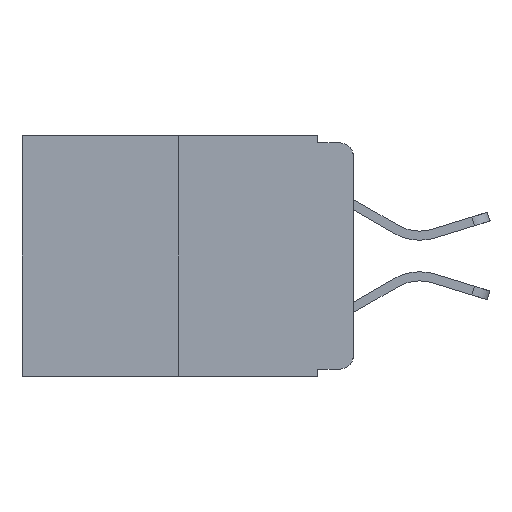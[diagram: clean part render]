
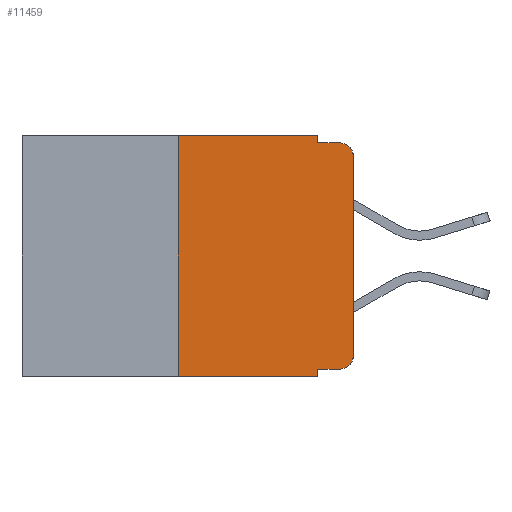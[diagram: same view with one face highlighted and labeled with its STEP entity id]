
A CAD part, left-side view. The second image highlights one B-rep face of the part: STEP entity #11459.
In plain terms, the highlighted planar face has unit normal (-1, 0, 0).
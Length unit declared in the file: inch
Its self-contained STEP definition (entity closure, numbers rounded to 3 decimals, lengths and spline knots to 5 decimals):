
#16 = ORIENTED_EDGE ( 'NONE', *, *, #14934, .T. ) ;
#308 = CARTESIAN_POINT ( 'NONE',  ( 0., 0.473, -0.343 ) ) ;
#484 = VERTEX_POINT ( 'NONE', #1440 ) ;
#561 = ORIENTED_EDGE ( 'NONE', *, *, #11764, .T. ) ;
#625 = VERTEX_POINT ( 'NONE', #16814 ) ;
#957 = VERTEX_POINT ( 'NONE', #11274 ) ;
#1167 = DIRECTION ( 'NONE',  ( 0., -1., 0. ) ) ;
#1254 = DIRECTION ( 'NONE',  ( 0., 0., -1. ) ) ;
#1336 = CARTESIAN_POINT ( 'NONE',  ( 0., 0., -0.03 ) ) ;
#1440 = CARTESIAN_POINT ( 'NONE',  ( 0., 0.25, 0. ) ) ;
#1723 = LINE ( 'NONE', #308, #2253 ) ;
#1852 = DIRECTION ( 'NONE',  ( 0., 0., 1. ) ) ;
#2253 = VECTOR ( 'NONE', #12218, 39.37008 ) ;
#2530 = LINE ( 'NONE', #21416, #11061 ) ;
#2687 = DIRECTION ( 'NONE',  ( -1., 0., 0. ) ) ;
#2775 = VERTEX_POINT ( 'NONE', #3604 ) ;
#3327 = AXIS2_PLACEMENT_3D ( 'NONE', #12826, #2687, #14473 ) ;
#3355 = CARTESIAN_POINT ( 'NONE',  ( 0., 0.473, 0. ) ) ;
#3604 = CARTESIAN_POINT ( 'NONE',  ( 0., 0.02, -0.01 ) ) ;
#3708 = LINE ( 'NONE', #10699, #19916 ) ;
#4062 = VECTOR ( 'NONE', #1254, 39.37008 ) ;
#4290 = EDGE_CURVE ( 'NONE', #8456, #625, #13938, .T. ) ;
#4429 = VECTOR ( 'NONE', #21530, 39.37008 ) ;
#4497 = VERTEX_POINT ( 'NONE', #16687 ) ;
#4848 = ORIENTED_EDGE ( 'NONE', *, *, #7164, .F. ) ;
#4855 = CARTESIAN_POINT ( 'NONE',  ( 0., 0.02, -0.333 ) ) ;
#5078 = DIRECTION ( 'NONE',  ( 0., 0., -1. ) ) ;
#5144 = CARTESIAN_POINT ( 'NONE',  ( 0., 0.051, -0.343 ) ) ;
#5331 = EDGE_CURVE ( 'NONE', #4497, #6767, #1723, .T. ) ;
#5655 = DIRECTION ( 'NONE',  ( 0., -1., 0. ) ) ;
#6253 = CARTESIAN_POINT ( 'NONE',  ( 0., 0.051, -0.01 ) ) ;
#6574 = EDGE_CURVE ( 'NONE', #21223, #2775, #9388, .T. ) ;
#6767 = VERTEX_POINT ( 'NONE', #5144 ) ;
#7164 = EDGE_CURVE ( 'NONE', #19068, #21223, #2530, .T. ) ;
#7581 = LINE ( 'NONE', #10331, #11558 ) ;
#8456 = VERTEX_POINT ( 'NONE', #4855 ) ;
#8592 = AXIS2_PLACEMENT_3D ( 'NONE', #3355, #15080, #5078 ) ;
#9197 = AXIS2_PLACEMENT_3D ( 'NONE', #9633, #21211, #11357 ) ;
#9286 = EDGE_CURVE ( 'NONE', #957, #6767, #17385, .T. ) ;
#9320 = ORIENTED_EDGE ( 'NONE', *, *, #14581, .F. ) ;
#9388 = LINE ( 'NONE', #6253, #14837 ) ;
#9457 = ORIENTED_EDGE ( 'NONE', *, *, #13046, .T. ) ;
#9633 = CARTESIAN_POINT ( 'NONE',  ( 0., 0.02, -0.03 ) ) ;
#10331 = CARTESIAN_POINT ( 'NONE',  ( 0., 0.25, 0. ) ) ;
#10699 = CARTESIAN_POINT ( 'NONE',  ( 0., 0.473, 0. ) ) ;
#10970 = ORIENTED_EDGE ( 'NONE', *, *, #6574, .F. ) ;
#11061 = VECTOR ( 'NONE', #14852, 39.37008 ) ;
#11274 = CARTESIAN_POINT ( 'NONE',  ( 0., 0.051, -0.333 ) ) ;
#11357 = DIRECTION ( 'NONE',  ( 0., 0., -1. ) ) ;
#11459 = ADVANCED_FACE ( 'NONE', ( #14244 ), #13460, .F. ) ;
#11558 = VECTOR ( 'NONE', #1852, 39.37008 ) ;
#11764 = EDGE_CURVE ( 'NONE', #625, #17745, #21182, .T. ) ;
#12218 = DIRECTION ( 'NONE',  ( 0., -1., 0. ) ) ;
#12447 = VECTOR ( 'NONE', #12943, 39.37008 ) ;
#12557 = ORIENTED_EDGE ( 'NONE', *, *, #9286, .F. ) ;
#12826 = CARTESIAN_POINT ( 'NONE',  ( 0., 0.02, -0.313 ) ) ;
#12943 = DIRECTION ( 'NONE',  ( 0., 0., 1. ) ) ;
#13046 = EDGE_CURVE ( 'NONE', #957, #8456, #13404, .T. ) ;
#13404 = LINE ( 'NONE', #19894, #4429 ) ;
#13460 = PLANE ( 'NONE',  #8592 ) ;
#13938 = CIRCLE ( 'NONE', #3327, 0.02 ) ;
#14244 = FACE_OUTER_BOUND ( 'NONE', #21684, .T. ) ;
#14473 = DIRECTION ( 'NONE',  ( 0., 0., -1. ) ) ;
#14522 = CARTESIAN_POINT ( 'NONE',  ( 0., 0., 0. ) ) ;
#14581 = EDGE_CURVE ( 'NONE', #4497, #484, #7581, .T. ) ;
#14837 = VECTOR ( 'NONE', #1167, 39.37008 ) ;
#14852 = DIRECTION ( 'NONE',  ( 0., 0., -1. ) ) ;
#14934 = EDGE_CURVE ( 'NONE', #17745, #2775, #17969, .T. ) ;
#15034 = ORIENTED_EDGE ( 'NONE', *, *, #18615, .F. ) ;
#15080 = DIRECTION ( 'NONE',  ( 1., 0., 0. ) ) ;
#15912 = ORIENTED_EDGE ( 'NONE', *, *, #5331, .T. ) ;
#16687 = CARTESIAN_POINT ( 'NONE',  ( 0., 0.25, -0.343 ) ) ;
#16777 = CARTESIAN_POINT ( 'NONE',  ( 0., 0.051, -0.01 ) ) ;
#16814 = CARTESIAN_POINT ( 'NONE',  ( 0., 0., -0.313 ) ) ;
#17385 = LINE ( 'NONE', #21321, #4062 ) ;
#17745 = VERTEX_POINT ( 'NONE', #1336 ) ;
#17969 = CIRCLE ( 'NONE', #9197, 0.02 ) ;
#18549 = CARTESIAN_POINT ( 'NONE',  ( 0., 0.051, 0. ) ) ;
#18565 = ORIENTED_EDGE ( 'NONE', *, *, #4290, .T. ) ;
#18615 = EDGE_CURVE ( 'NONE', #484, #19068, #3708, .T. ) ;
#19068 = VERTEX_POINT ( 'NONE', #18549 ) ;
#19894 = CARTESIAN_POINT ( 'NONE',  ( 0., 0.051, -0.333 ) ) ;
#19916 = VECTOR ( 'NONE', #5655, 39.37008 ) ;
#21182 = LINE ( 'NONE', #14522, #12447 ) ;
#21211 = DIRECTION ( 'NONE',  ( -1., 0., 0. ) ) ;
#21223 = VERTEX_POINT ( 'NONE', #16777 ) ;
#21321 = CARTESIAN_POINT ( 'NONE',  ( 0., 0.051, 0. ) ) ;
#21416 = CARTESIAN_POINT ( 'NONE',  ( 0., 0.051, 0. ) ) ;
#21530 = DIRECTION ( 'NONE',  ( 0., -1., 0. ) ) ;
#21684 = EDGE_LOOP ( 'NONE', ( #561, #16, #10970, #4848, #15034, #9320, #15912, #12557, #9457, #18565 ) ) ;
